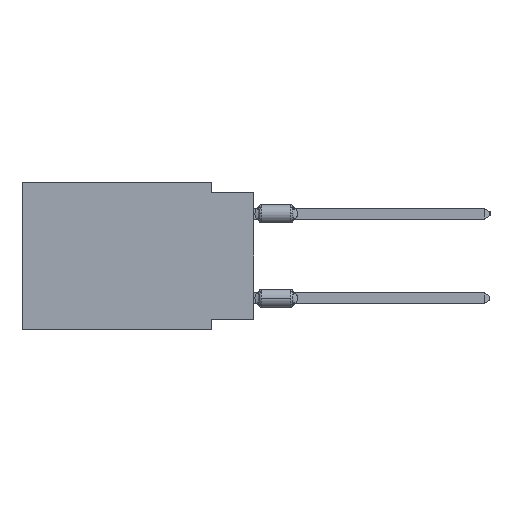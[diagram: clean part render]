
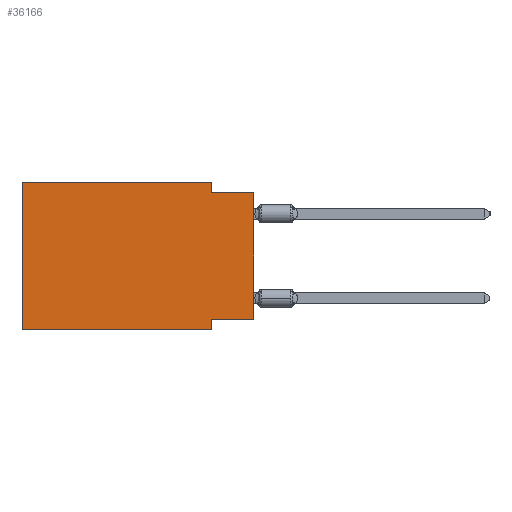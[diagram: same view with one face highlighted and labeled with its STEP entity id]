
A CAD part, left-side view. The second image highlights one B-rep face of the part: STEP entity #36166.
In plain terms, the highlighted planar face has unit normal (-1, 0, 0).
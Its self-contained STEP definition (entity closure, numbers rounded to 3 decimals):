
#1634 = VERTEX_POINT ( 'NONE', #30498 ) ;
#3112 = VECTOR ( 'NONE', #31988, 1000. ) ;
#3744 = CARTESIAN_POINT ( 'NONE',  ( 0., 2.54, -8.89 ) ) ;
#4832 = CARTESIAN_POINT ( 'NONE',  ( 0., 13.97, -8.89 ) ) ;
#5357 = ORIENTED_EDGE ( 'NONE', *, *, #29688, .F. ) ;
#6330 = CARTESIAN_POINT ( 'NONE',  ( 0., 13.97, 0. ) ) ;
#6531 = CARTESIAN_POINT ( 'NONE',  ( 0., 0., -0.635 ) ) ;
#9126 = CARTESIAN_POINT ( 'NONE',  ( 0., 2.54, 0. ) ) ;
#9651 = CARTESIAN_POINT ( 'NONE',  ( 0., 13.97, 0. ) ) ;
#11944 = AXIS2_PLACEMENT_3D ( 'NONE', #6330, #26554, #38410 ) ;
#13463 = ORIENTED_EDGE ( 'NONE', *, *, #41242, .F. ) ;
#14313 = EDGE_CURVE ( 'NONE', #21823, #32194, #57786, .T. ) ;
#20228 = CARTESIAN_POINT ( 'NONE',  ( 0., 2.54, -8.255 ) ) ;
#21823 = VERTEX_POINT ( 'NONE', #36878 ) ;
#21891 = DIRECTION ( 'NONE',  ( 0., -1., 0. ) ) ;
#21920 = ORIENTED_EDGE ( 'NONE', *, *, #54686, .F. ) ;
#22130 = LINE ( 'NONE', #43390, #66872 ) ;
#26554 = DIRECTION ( 'NONE',  ( 1., 0., 0. ) ) ;
#26906 = PLANE ( 'NONE',  #11944 ) ;
#27749 = EDGE_CURVE ( 'NONE', #64863, #42724, #22130, .T. ) ;
#27794 = DIRECTION ( 'NONE',  ( 0., -1., 0. ) ) ;
#28822 = CARTESIAN_POINT ( 'NONE',  ( 0., 2.54, -8.89 ) ) ;
#29688 = EDGE_CURVE ( 'NONE', #62675, #42724, #54267, .T. ) ;
#30498 = CARTESIAN_POINT ( 'NONE',  ( 0., 13.97, 0. ) ) ;
#30600 = EDGE_CURVE ( 'NONE', #65356, #32194, #34057, .T. ) ;
#30833 = CARTESIAN_POINT ( 'NONE',  ( 0., 0., -8.255 ) ) ;
#30957 = CARTESIAN_POINT ( 'NONE',  ( 0., 13.97, 0. ) ) ;
#31988 = DIRECTION ( 'NONE',  ( 0., -1., 0. ) ) ;
#32194 = VERTEX_POINT ( 'NONE', #3744 ) ;
#32377 = DIRECTION ( 'NONE',  ( 0., 1., 0. ) ) ;
#34057 = LINE ( 'NONE', #28822, #50358 ) ;
#35945 = DIRECTION ( 'NONE',  ( 0., 0., -1. ) ) ;
#36166 = ADVANCED_FACE ( 'NONE', ( #53370 ), #26906, .F. ) ;
#36831 = VECTOR ( 'NONE', #35945, 1000. ) ;
#36878 = CARTESIAN_POINT ( 'NONE',  ( 0., 13.97, -8.89 ) ) ;
#37690 = VECTOR ( 'NONE', #21891, 1000. ) ;
#37708 = ORIENTED_EDGE ( 'NONE', *, *, #14313, .T. ) ;
#38410 = DIRECTION ( 'NONE',  ( 0., 0., -1. ) ) ;
#38874 = CARTESIAN_POINT ( 'NONE',  ( 0., 2.54, 0. ) ) ;
#39283 = VECTOR ( 'NONE', #27794, 1000. ) ;
#39972 = CARTESIAN_POINT ( 'NONE',  ( 0., 0., -0.635 ) ) ;
#40186 = LINE ( 'NONE', #9126, #36831 ) ;
#40206 = EDGE_LOOP ( 'NONE', ( #51578, #5357, #49819, #21920, #13463, #37708, #59970, #43091 ) ) ;
#41242 = EDGE_CURVE ( 'NONE', #21823, #1634, #57720, .T. ) ;
#42724 = VERTEX_POINT ( 'NONE', #39972 ) ;
#43091 = ORIENTED_EDGE ( 'NONE', *, *, #64166, .F. ) ;
#43390 = CARTESIAN_POINT ( 'NONE',  ( 0., 0., 0. ) ) ;
#44256 = EDGE_CURVE ( 'NONE', #68063, #62675, #40186, .T. ) ;
#47021 = VECTOR ( 'NONE', #32377, 1000. ) ;
#49819 = ORIENTED_EDGE ( 'NONE', *, *, #44256, .F. ) ;
#50071 = DIRECTION ( 'NONE',  ( 0., 0., -1. ) ) ;
#50358 = VECTOR ( 'NONE', #50071, 1000. ) ;
#51578 = ORIENTED_EDGE ( 'NONE', *, *, #27749, .T. ) ;
#52210 = LINE ( 'NONE', #30957, #3112 ) ;
#53370 = FACE_OUTER_BOUND ( 'NONE', #40206, .T. ) ;
#54267 = LINE ( 'NONE', #6531, #39283 ) ;
#54501 = VECTOR ( 'NONE', #63972, 1000. ) ;
#54686 = EDGE_CURVE ( 'NONE', #1634, #68063, #52210, .T. ) ;
#57720 = LINE ( 'NONE', #9651, #54501 ) ;
#57786 = LINE ( 'NONE', #4832, #37690 ) ;
#59202 = CARTESIAN_POINT ( 'NONE',  ( 0., 0., -8.255 ) ) ;
#59970 = ORIENTED_EDGE ( 'NONE', *, *, #30600, .F. ) ;
#62675 = VERTEX_POINT ( 'NONE', #65835 ) ;
#63972 = DIRECTION ( 'NONE',  ( 0., 0., 1. ) ) ;
#64166 = EDGE_CURVE ( 'NONE', #64863, #65356, #64418, .T. ) ;
#64418 = LINE ( 'NONE', #59202, #47021 ) ;
#64863 = VERTEX_POINT ( 'NONE', #30833 ) ;
#64984 = DIRECTION ( 'NONE',  ( 0., 0., 1. ) ) ;
#65356 = VERTEX_POINT ( 'NONE', #20228 ) ;
#65835 = CARTESIAN_POINT ( 'NONE',  ( 0., 2.54, -0.635 ) ) ;
#66872 = VECTOR ( 'NONE', #64984, 1000. ) ;
#68063 = VERTEX_POINT ( 'NONE', #38874 ) ;
